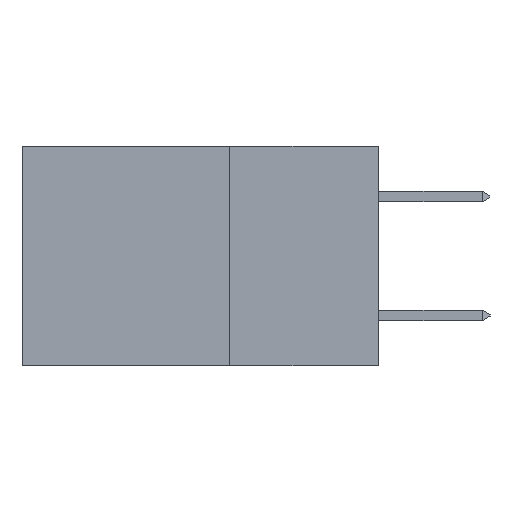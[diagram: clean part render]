
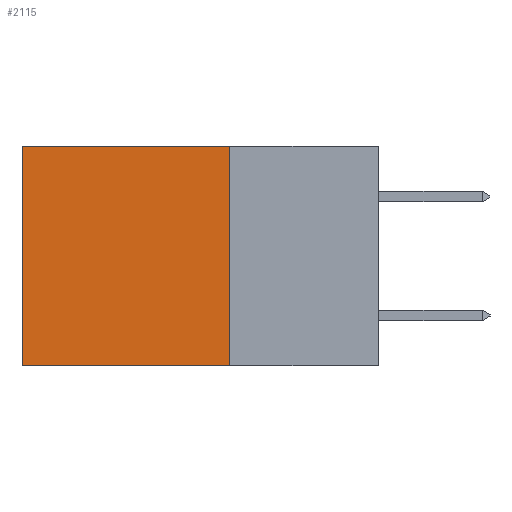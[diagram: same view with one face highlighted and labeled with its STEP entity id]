
A CAD part, left-side view. The second image highlights one B-rep face of the part: STEP entity #2115.
In plain terms, the highlighted planar face has unit normal (-1, 0, 0).
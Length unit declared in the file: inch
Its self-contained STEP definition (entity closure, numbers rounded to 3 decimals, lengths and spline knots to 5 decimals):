
#159 = VERTEX_POINT ( 'NONE', #1084 ) ;
#241 = VECTOR ( 'NONE', #3318, 39.37008 ) ;
#831 = CARTESIAN_POINT ( 'NONE',  ( 0.2615, 0.25, -0.37 ) ) ;
#886 = EDGE_LOOP ( 'NONE', ( #16896, #5559, #3175, #12461 ) ) ;
#1084 = CARTESIAN_POINT ( 'NONE',  ( 0.2615, 0.25, -0.37 ) ) ;
#2115 = ADVANCED_FACE ( 'NONE', ( #11806 ), #12424, .F. ) ;
#2702 = VECTOR ( 'NONE', #11284, 39.37008 ) ;
#3175 = ORIENTED_EDGE ( 'NONE', *, *, #7490, .F. ) ;
#3318 = DIRECTION ( 'NONE',  ( 0., 0., -1. ) ) ;
#4233 = AXIS2_PLACEMENT_3D ( 'NONE', #831, #8718, #13369 ) ;
#4368 = LINE ( 'NONE', #17085, #241 ) ;
#4703 = VECTOR ( 'NONE', #6470, 39.37008 ) ;
#5559 = ORIENTED_EDGE ( 'NONE', *, *, #13195, .F. ) ;
#6470 = DIRECTION ( 'NONE',  ( 0., 1., 0. ) ) ;
#7490 = EDGE_CURVE ( 'NONE', #8852, #159, #17606, .T. ) ;
#8718 = DIRECTION ( 'NONE',  ( 1., 0., 0. ) ) ;
#8852 = VERTEX_POINT ( 'NONE', #11526 ) ;
#9237 = DIRECTION ( 'NONE',  ( 0., 0., -1. ) ) ;
#9241 = CARTESIAN_POINT ( 'NONE',  ( 0.2615, 0.25, -0.37 ) ) ;
#11284 = DIRECTION ( 'NONE',  ( 0., 1., 0. ) ) ;
#11526 = CARTESIAN_POINT ( 'NONE',  ( 0.2615, 0.25, 0. ) ) ;
#11806 = FACE_OUTER_BOUND ( 'NONE', #886, .T. ) ;
#12424 = PLANE ( 'NONE',  #4233 ) ;
#12461 = ORIENTED_EDGE ( 'NONE', *, *, #12867, .T. ) ;
#12466 = LINE ( 'NONE', #16074, #4703 ) ;
#12501 = VERTEX_POINT ( 'NONE', #13991 ) ;
#12867 = EDGE_CURVE ( 'NONE', #8852, #12501, #12466, .T. ) ;
#13195 = EDGE_CURVE ( 'NONE', #159, #17678, #14186, .T. ) ;
#13369 = DIRECTION ( 'NONE',  ( 0., 0., -1. ) ) ;
#13991 = CARTESIAN_POINT ( 'NONE',  ( 0.2615, 0.6, 0. ) ) ;
#14030 = CARTESIAN_POINT ( 'NONE',  ( 0.2615, 0.25, -0.37 ) ) ;
#14186 = LINE ( 'NONE', #14030, #2702 ) ;
#15285 = EDGE_CURVE ( 'NONE', #12501, #17678, #4368, .T. ) ;
#16074 = CARTESIAN_POINT ( 'NONE',  ( 0.2615, 0.25, 0. ) ) ;
#16848 = CARTESIAN_POINT ( 'NONE',  ( 0.2615, 0.6, -0.37 ) ) ;
#16896 = ORIENTED_EDGE ( 'NONE', *, *, #15285, .T. ) ;
#17085 = CARTESIAN_POINT ( 'NONE',  ( 0.2615, 0.6, -0.37 ) ) ;
#17198 = VECTOR ( 'NONE', #9237, 39.37008 ) ;
#17606 = LINE ( 'NONE', #9241, #17198 ) ;
#17678 = VERTEX_POINT ( 'NONE', #16848 ) ;
